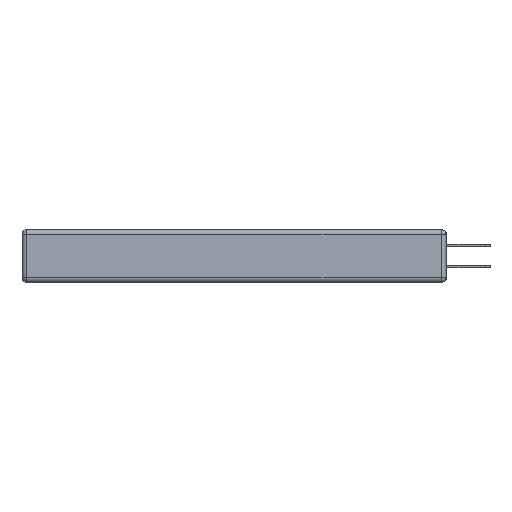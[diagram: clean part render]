
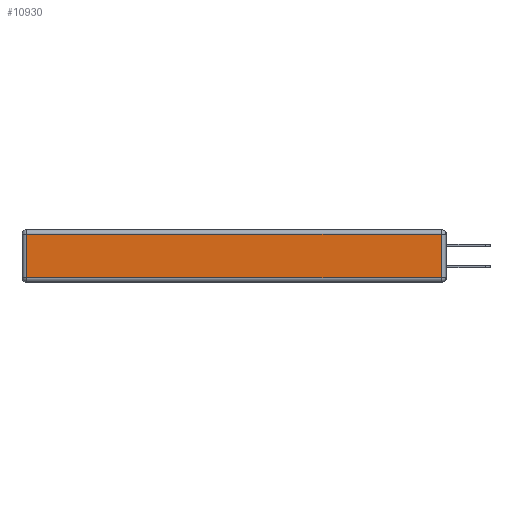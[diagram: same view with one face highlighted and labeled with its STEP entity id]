
A CAD part, left-side view. The second image highlights one B-rep face of the part: STEP entity #10930.
In plain terms, the highlighted planar face has unit normal (-1, 0, 0).
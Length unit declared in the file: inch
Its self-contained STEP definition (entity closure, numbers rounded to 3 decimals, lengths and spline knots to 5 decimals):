
#43 = DIRECTION ( 'NONE',  ( 0., 1., 0. ) ) ;
#123 = LINE ( 'NONE', #4969, #4096 ) ;
#304 = DIRECTION ( 'NONE',  ( 0., -1., 0. ) ) ;
#868 = ORIENTED_EDGE ( 'NONE', *, *, #3738, .T. ) ;
#936 = ORIENTED_EDGE ( 'NONE', *, *, #8004, .T. ) ;
#1075 = VERTEX_POINT ( 'NONE', #15120 ) ;
#1349 = ORIENTED_EDGE ( 'NONE', *, *, #1750, .T. ) ;
#1750 = EDGE_CURVE ( 'NONE', #1075, #10607, #13918, .T. ) ;
#1790 = VECTOR ( 'NONE', #7275, 39.37008 ) ;
#3184 = LINE ( 'NONE', #12552, #1790 ) ;
#3260 = EDGE_LOOP ( 'NONE', ( #868, #1349, #936, #7109 ) ) ;
#3628 = FACE_OUTER_BOUND ( 'NONE', #3260, .T. ) ;
#3738 = EDGE_CURVE ( 'NONE', #11322, #1075, #14834, .T. ) ;
#4096 = VECTOR ( 'NONE', #43, 39.37008 ) ;
#4969 = CARTESIAN_POINT ( 'NONE',  ( 0., 2.75, -0.03 ) ) ;
#5463 = VECTOR ( 'NONE', #304, 39.37008 ) ;
#5529 = DIRECTION ( 'NONE',  ( 0., 0., 1. ) ) ;
#6147 = EDGE_CURVE ( 'NONE', #14611, #11322, #3184, .T. ) ;
#7109 = ORIENTED_EDGE ( 'NONE', *, *, #6147, .T. ) ;
#7275 = DIRECTION ( 'NONE',  ( 0., 0., -1. ) ) ;
#7962 = CARTESIAN_POINT ( 'NONE',  ( 0., 0., -0.313 ) ) ;
#8004 = EDGE_CURVE ( 'NONE', #10607, #14611, #123, .T. ) ;
#9280 = CARTESIAN_POINT ( 'NONE',  ( 0., 0.03, -0.03 ) ) ;
#10607 = VERTEX_POINT ( 'NONE', #9280 ) ;
#10930 = ADVANCED_FACE ( 'NONE', ( #3628 ), #15222, .T. ) ;
#11322 = VERTEX_POINT ( 'NONE', #14722 ) ;
#11369 = DIRECTION ( 'NONE',  ( -1., 0., 0. ) ) ;
#11721 = CARTESIAN_POINT ( 'NONE',  ( 0., 2.72, -0.03 ) ) ;
#11868 = CARTESIAN_POINT ( 'NONE',  ( 0., 0.03, -0.343 ) ) ;
#12520 = DIRECTION ( 'NONE',  ( 0., 0., 1. ) ) ;
#12552 = CARTESIAN_POINT ( 'NONE',  ( 0., 2.72, -0.343 ) ) ;
#13352 = VECTOR ( 'NONE', #5529, 39.37008 ) ;
#13918 = LINE ( 'NONE', #11868, #13352 ) ;
#14611 = VERTEX_POINT ( 'NONE', #11721 ) ;
#14722 = CARTESIAN_POINT ( 'NONE',  ( 0., 2.72, -0.313 ) ) ;
#14834 = LINE ( 'NONE', #7962, #5463 ) ;
#15120 = CARTESIAN_POINT ( 'NONE',  ( 0., 0.03, -0.313 ) ) ;
#15222 = PLANE ( 'NONE',  #16497 ) ;
#16368 = CARTESIAN_POINT ( 'NONE',  ( 0., 0., -0.343 ) ) ;
#16497 = AXIS2_PLACEMENT_3D ( 'NONE', #16368, #11369, #12520 ) ;
